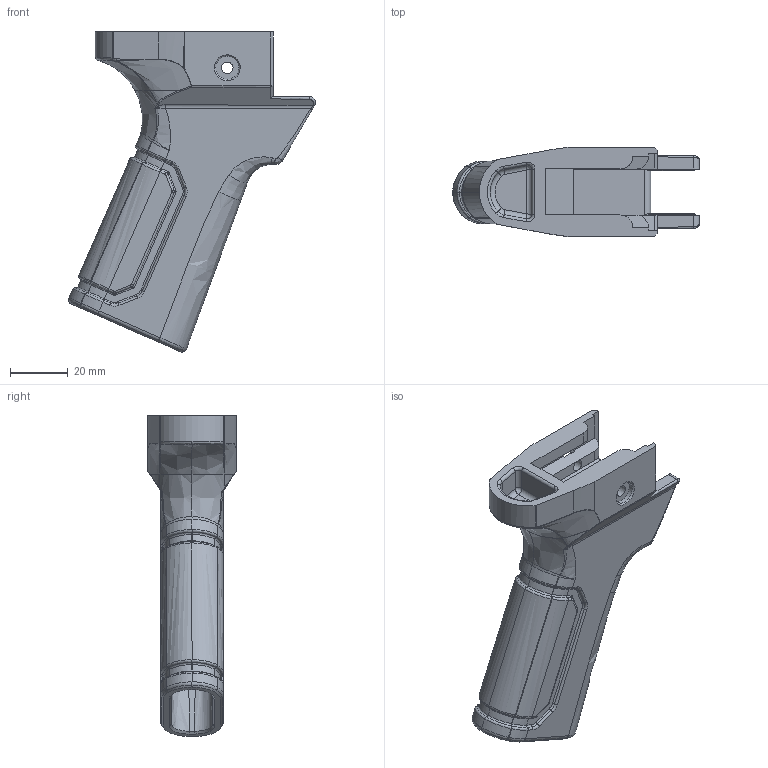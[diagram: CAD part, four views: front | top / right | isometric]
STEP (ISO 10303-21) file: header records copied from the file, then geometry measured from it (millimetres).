
FILE_DESCRIPTION(/* description */ (''),/* implementation_level */ '2;1');
FILE_NAME(/* name */ 'Padded Grip.step',/* time_stamp */ '2021-08-26T02:23:52-04:00',/* author */ (''),/* organization */ (''),/* preprocessor_version */ 'ST-DEVELOPER v18.1',/* originating_system */ 'Autodesk Translation Framework v10.10.0.1391',/* authorisation */ '');
FILE_SCHEMA (('AUTOMOTIVE_DESIGN { 1 0 10303 214 3 1 1 }'));
Length unit declared in the file: millimetre
Products named in the file (1): Padded Grip
Bounding box: 85.78 x 31 x 111.55 mm (x, y, z)
Volume: 58172.7 mm3; surface area: 26942.9 mm2
Topology: 1 solids, 1 shells, 510 faces, 1278 edges, 747 vertices
Faces by surface type: bspline 250, plane 102, cylinder 97, torus 44, sphere 14, cone 3
Full cylindrical faces by diameter (mm): 4 x2, 8 x1
Entity records: 27852 total; most frequent: CARTESIAN_POINT 17358, ORIENTED_EDGE 2506, DIRECTION 1638, EDGE_CURVE 1253, VERTEX_POINT 747, AXIS2_PLACEMENT_3D 637, EDGE_LOOP 520, B_SPLINE_CURVE_WITH_KNOTS 513
